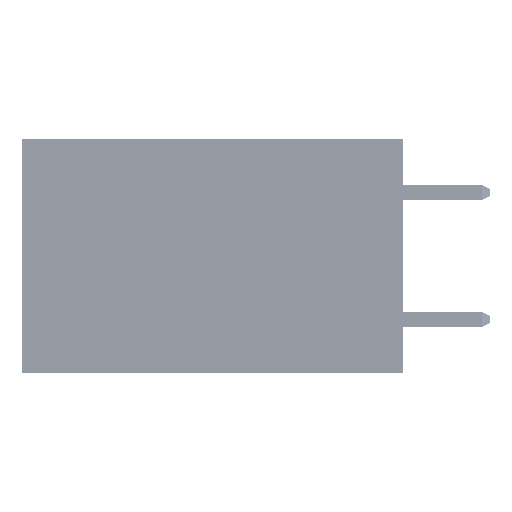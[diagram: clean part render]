
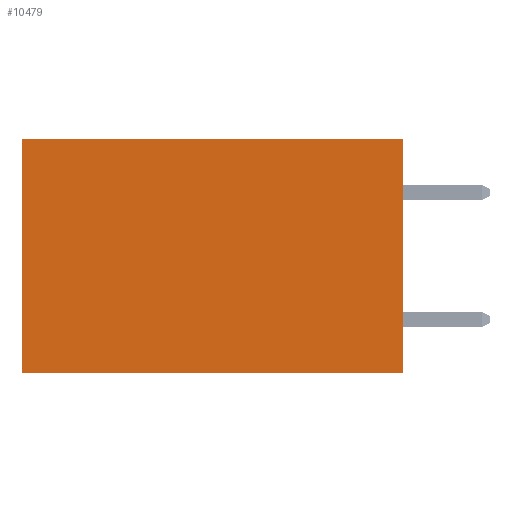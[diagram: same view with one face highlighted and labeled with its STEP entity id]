
A CAD part, left-side view. The second image highlights one B-rep face of the part: STEP entity #10479.
In plain terms, the highlighted planar face has unit normal (-1, 0, 0).
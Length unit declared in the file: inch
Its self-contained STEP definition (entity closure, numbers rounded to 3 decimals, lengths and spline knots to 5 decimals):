
#2280 = DIRECTION ( 'NONE',  ( 0., 0., -1. ) ) ;
#3264 = CARTESIAN_POINT ( 'NONE',  ( 0.2875, 0., -0.37 ) ) ;
#4753 = EDGE_CURVE ( 'NONE', #38853, #19771, #42557, .T. ) ;
#5267 = AXIS2_PLACEMENT_3D ( 'NONE', #13837, #47397, #2280 ) ;
#6617 = CARTESIAN_POINT ( 'NONE',  ( 0.2875, 0., 0. ) ) ;
#7113 = ORIENTED_EDGE ( 'NONE', *, *, #4753, .F. ) ;
#7149 = DIRECTION ( 'NONE',  ( 0., 1., 0. ) ) ;
#7360 = EDGE_LOOP ( 'NONE', ( #32845, #7113, #8215, #24302 ) ) ;
#8215 = ORIENTED_EDGE ( 'NONE', *, *, #42955, .F. ) ;
#9122 = CARTESIAN_POINT ( 'NONE',  ( 0.2875, 0., -0.37 ) ) ;
#9298 = DIRECTION ( 'NONE',  ( 0., 1., 0. ) ) ;
#10479 = ADVANCED_FACE ( 'NONE', ( #12504 ), #20694, .F. ) ;
#11816 = VECTOR ( 'NONE', #28734, 39.37008 ) ;
#12008 = EDGE_CURVE ( 'NONE', #26526, #19771, #14142, .T. ) ;
#12504 = FACE_OUTER_BOUND ( 'NONE', #7360, .T. ) ;
#13219 = LINE ( 'NONE', #20561, #25504 ) ;
#13837 = CARTESIAN_POINT ( 'NONE',  ( 0.2875, 0., 0. ) ) ;
#14142 = LINE ( 'NONE', #47603, #11816 ) ;
#16293 = VECTOR ( 'NONE', #7149, 39.37008 ) ;
#19093 = EDGE_CURVE ( 'NONE', #30769, #26526, #13219, .T. ) ;
#19771 = VERTEX_POINT ( 'NONE', #32388 ) ;
#20561 = CARTESIAN_POINT ( 'NONE',  ( 0.2875, 0., 0. ) ) ;
#20694 = PLANE ( 'NONE',  #5267 ) ;
#23225 = CARTESIAN_POINT ( 'NONE',  ( 0.2875, 0.6, 0. ) ) ;
#24302 = ORIENTED_EDGE ( 'NONE', *, *, #19093, .T. ) ;
#25504 = VECTOR ( 'NONE', #9298, 39.37008 ) ;
#26526 = VERTEX_POINT ( 'NONE', #23225 ) ;
#27706 = LINE ( 'NONE', #37480, #44596 ) ;
#28734 = DIRECTION ( 'NONE',  ( 0., 0., -1. ) ) ;
#30769 = VERTEX_POINT ( 'NONE', #6617 ) ;
#32388 = CARTESIAN_POINT ( 'NONE',  ( 0.2875, 0.6, -0.37 ) ) ;
#32845 = ORIENTED_EDGE ( 'NONE', *, *, #12008, .T. ) ;
#37480 = CARTESIAN_POINT ( 'NONE',  ( 0.2875, 0., 0. ) ) ;
#38853 = VERTEX_POINT ( 'NONE', #9122 ) ;
#42557 = LINE ( 'NONE', #3264, #16293 ) ;
#42955 = EDGE_CURVE ( 'NONE', #30769, #38853, #27706, .T. ) ;
#44596 = VECTOR ( 'NONE', #45325, 39.37008 ) ;
#45325 = DIRECTION ( 'NONE',  ( 0., 0., -1. ) ) ;
#47397 = DIRECTION ( 'NONE',  ( 1., 0., 0. ) ) ;
#47603 = CARTESIAN_POINT ( 'NONE',  ( 0.2875, 0.6, 0. ) ) ;
